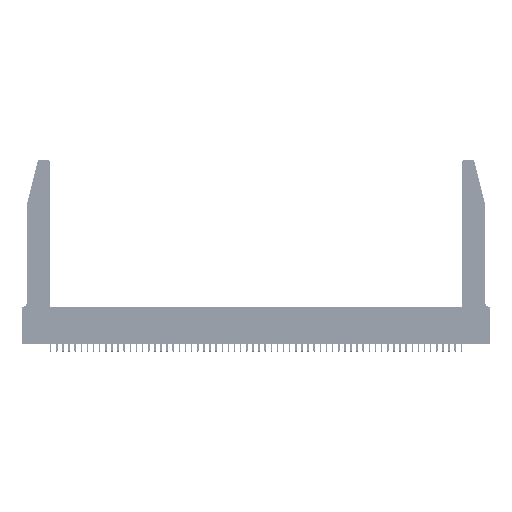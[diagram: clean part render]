
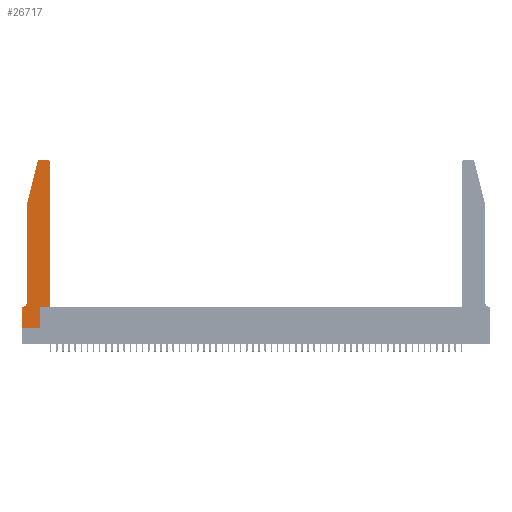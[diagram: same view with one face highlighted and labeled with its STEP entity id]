
A CAD part, top view. The second image highlights one B-rep face of the part: STEP entity #26717.
In plain terms, the highlighted planar face has unit normal (0, 0, 1).
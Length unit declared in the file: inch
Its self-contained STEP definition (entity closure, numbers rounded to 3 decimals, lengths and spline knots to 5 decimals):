
#347 = DIRECTION ( 'NONE',  ( -1., 0., 0. ) ) ;
#642 = LINE ( 'NONE', #931, #15140 ) ;
#931 = CARTESIAN_POINT ( 'NONE',  ( 0., 0., 0.37 ) ) ;
#1450 = VERTEX_POINT ( 'NONE', #10823 ) ;
#2119 = ORIENTED_EDGE ( 'NONE', *, *, #18307, .T. ) ;
#3157 = VECTOR ( 'NONE', #11315, 39.37008 ) ;
#3925 = AXIS2_PLACEMENT_3D ( 'NONE', #12461, #20213, #28775 ) ;
#4512 = ORIENTED_EDGE ( 'NONE', *, *, #24507, .T. ) ;
#5059 = VERTEX_POINT ( 'NONE', #45349 ) ;
#6783 = CARTESIAN_POINT ( 'NONE',  ( 0.4505, 0.35, 0.37 ) ) ;
#7044 = PLANE ( 'NONE',  #51163 ) ;
#7234 = CARTESIAN_POINT ( 'NONE',  ( 0.0755, 0.42, 0.37 ) ) ;
#7421 = CARTESIAN_POINT ( 'NONE',  ( 0.2605, 2.75, 0.37 ) ) ;
#7817 = ORIENTED_EDGE ( 'NONE', *, *, #23301, .T. ) ;
#8553 = DIRECTION ( 'NONE',  ( 0., -1., 0. ) ) ;
#9873 = VERTEX_POINT ( 'NONE', #6783 ) ;
#9878 = VECTOR ( 'NONE', #52754, 39.37008 ) ;
#10526 = CARTESIAN_POINT ( 'NONE',  ( 0.4505, 0.35, 0.37 ) ) ;
#10560 = ORIENTED_EDGE ( 'NONE', *, *, #50971, .T. ) ;
#10823 = CARTESIAN_POINT ( 'NONE',  ( 0.4205, 2.75, 0.37 ) ) ;
#10833 = CARTESIAN_POINT ( 'NONE',  ( 0., 0., 0.37 ) ) ;
#11045 = LINE ( 'NONE', #17333, #48696 ) ;
#11091 = ORIENTED_EDGE ( 'NONE', *, *, #27144, .T. ) ;
#11315 = DIRECTION ( 'NONE',  ( -1., 0., 0. ) ) ;
#12461 = CARTESIAN_POINT ( 'NONE',  ( 0.4205, 2.72, 0.37 ) ) ;
#13019 = CARTESIAN_POINT ( 'NONE',  ( 0.284, 2.72, 0.37 ) ) ;
#13283 = DIRECTION ( 'NONE',  ( 0., 0., -1. ) ) ;
#13637 = EDGE_LOOP ( 'NONE', ( #4512, #51916, #36379, #36044, #37924, #2119, #11091, #45557, #10560, #7817, #50118, #32445 ) ) ;
#13944 = EDGE_CURVE ( 'NONE', #47232, #5059, #19849, .T. ) ;
#14658 = VERTEX_POINT ( 'NONE', #53064 ) ;
#15140 = VECTOR ( 'NONE', #43229, 39.37008 ) ;
#15670 = LINE ( 'NONE', #7421, #3157 ) ;
#16266 = EDGE_CURVE ( 'NONE', #21307, #50506, #31699, .T. ) ;
#16562 = VECTOR ( 'NONE', #36061, 39.37008 ) ;
#16847 = AXIS2_PLACEMENT_3D ( 'NONE', #25661, #13283, #347 ) ;
#16972 = CIRCLE ( 'NONE', #54122, 0.03 ) ;
#17333 = CARTESIAN_POINT ( 'NONE',  ( 0., 0., 0.37 ) ) ;
#17369 = CARTESIAN_POINT ( 'NONE',  ( 0.0755, 2., 0.37 ) ) ;
#18307 = EDGE_CURVE ( 'NONE', #50506, #20559, #40983, .T. ) ;
#18642 = CARTESIAN_POINT ( 'NONE',  ( 0.0755, 2., 0.37 ) ) ;
#19110 = CARTESIAN_POINT ( 'NONE',  ( 0.25487, 2.72718, 0.37 ) ) ;
#19638 = LINE ( 'NONE', #40955, #26958 ) ;
#19849 = LINE ( 'NONE', #18642, #16562 ) ;
#20213 = DIRECTION ( 'NONE',  ( 0., 0., 1. ) ) ;
#20559 = VERTEX_POINT ( 'NONE', #28203 ) ;
#21307 = VERTEX_POINT ( 'NONE', #7234 ) ;
#21331 = DIRECTION ( 'NONE',  ( -1., 0., 0. ) ) ;
#22280 = CARTESIAN_POINT ( 'NONE',  ( 0.2865, 0.35, 0.37 ) ) ;
#23301 = EDGE_CURVE ( 'NONE', #39117, #9873, #36360, .T. ) ;
#24507 = EDGE_CURVE ( 'NONE', #1450, #25675, #15670, .T. ) ;
#24852 = EDGE_CURVE ( 'NONE', #39287, #54596, #642, .T. ) ;
#25661 = CARTESIAN_POINT ( 'NONE',  ( 0.0055, 0.42, 0.37 ) ) ;
#25675 = VERTEX_POINT ( 'NONE', #53410 ) ;
#26146 = CIRCLE ( 'NONE', #3925, 0.03 ) ;
#26190 = CARTESIAN_POINT ( 'NONE',  ( 0.0755, 0.35, 0.37 ) ) ;
#26427 = DIRECTION ( 'NONE',  ( 0., -1., 0. ) ) ;
#26487 = VECTOR ( 'NONE', #21331, 39.37008 ) ;
#26717 = ADVANCED_FACE ( 'NONE', ( #46649 ), #7044, .T. ) ;
#26775 = LINE ( 'NONE', #17369, #52445 ) ;
#26958 = VECTOR ( 'NONE', #28427, 39.37008 ) ;
#27144 = EDGE_CURVE ( 'NONE', #20559, #39287, #11045, .T. ) ;
#28130 = DIRECTION ( 'NONE',  ( 1., 0., 0. ) ) ;
#28203 = CARTESIAN_POINT ( 'NONE',  ( 0., 0.35, 0.37 ) ) ;
#28427 = DIRECTION ( 'NONE',  ( 0., 1., 0. ) ) ;
#28775 = DIRECTION ( 'NONE',  ( 1., 0., 0. ) ) ;
#29474 = DIRECTION ( 'NONE',  ( 0., 1., 0. ) ) ;
#31301 = EDGE_CURVE ( 'NONE', #9873, #14658, #38681, .T. ) ;
#31699 = CIRCLE ( 'NONE', #16847, 0.07 ) ;
#32445 = ORIENTED_EDGE ( 'NONE', *, *, #42429, .T. ) ;
#33849 = EDGE_CURVE ( 'NONE', #5059, #21307, #26775, .T. ) ;
#36044 = ORIENTED_EDGE ( 'NONE', *, *, #33849, .T. ) ;
#36061 = DIRECTION ( 'NONE',  ( -0.239, -0.971, 0. ) ) ;
#36360 = LINE ( 'NONE', #10526, #9878 ) ;
#36379 = ORIENTED_EDGE ( 'NONE', *, *, #13944, .T. ) ;
#37360 = VECTOR ( 'NONE', #29474, 39.37008 ) ;
#37924 = ORIENTED_EDGE ( 'NONE', *, *, #16266, .T. ) ;
#37984 = DIRECTION ( 'NONE',  ( 0., 0., 1. ) ) ;
#38681 = LINE ( 'NONE', #46369, #37360 ) ;
#39001 = CARTESIAN_POINT ( 'NONE',  ( 0.2865, 0., 0.37 ) ) ;
#39117 = VERTEX_POINT ( 'NONE', #22280 ) ;
#39287 = VERTEX_POINT ( 'NONE', #10833 ) ;
#40491 = CARTESIAN_POINT ( 'NONE',  ( 0., 0.35, 0.37 ) ) ;
#40955 = CARTESIAN_POINT ( 'NONE',  ( 0.2865, 0.35, 0.37 ) ) ;
#40983 = LINE ( 'NONE', #26190, #26487 ) ;
#41541 = EDGE_CURVE ( 'NONE', #25675, #47232, #16972, .T. ) ;
#42387 = DIRECTION ( 'NONE',  ( 1., 0., 0. ) ) ;
#42429 = EDGE_CURVE ( 'NONE', #14658, #1450, #26146, .T. ) ;
#43229 = DIRECTION ( 'NONE',  ( 1., 0., 0. ) ) ;
#45349 = CARTESIAN_POINT ( 'NONE',  ( 0.0755, 2., 0.37 ) ) ;
#45557 = ORIENTED_EDGE ( 'NONE', *, *, #24852, .T. ) ;
#46369 = CARTESIAN_POINT ( 'NONE',  ( 0.4505, 0.35, 0.37 ) ) ;
#46649 = FACE_OUTER_BOUND ( 'NONE', #13637, .T. ) ;
#47232 = VERTEX_POINT ( 'NONE', #19110 ) ;
#48696 = VECTOR ( 'NONE', #26427, 39.37008 ) ;
#50118 = ORIENTED_EDGE ( 'NONE', *, *, #31301, .T. ) ;
#50506 = VERTEX_POINT ( 'NONE', #50622 ) ;
#50622 = CARTESIAN_POINT ( 'NONE',  ( 0.0055, 0.35, 0.37 ) ) ;
#50971 = EDGE_CURVE ( 'NONE', #54596, #39117, #19638, .T. ) ;
#51163 = AXIS2_PLACEMENT_3D ( 'NONE', #40491, #52982, #28130 ) ;
#51916 = ORIENTED_EDGE ( 'NONE', *, *, #41541, .T. ) ;
#52445 = VECTOR ( 'NONE', #8553, 39.37008 ) ;
#52754 = DIRECTION ( 'NONE',  ( 1., 0., 0. ) ) ;
#52982 = DIRECTION ( 'NONE',  ( 0., 0., 1. ) ) ;
#53064 = CARTESIAN_POINT ( 'NONE',  ( 0.4505, 2.72, 0.37 ) ) ;
#53410 = CARTESIAN_POINT ( 'NONE',  ( 0.284, 2.75, 0.37 ) ) ;
#54122 = AXIS2_PLACEMENT_3D ( 'NONE', #13019, #37984, #42387 ) ;
#54596 = VERTEX_POINT ( 'NONE', #39001 ) ;
